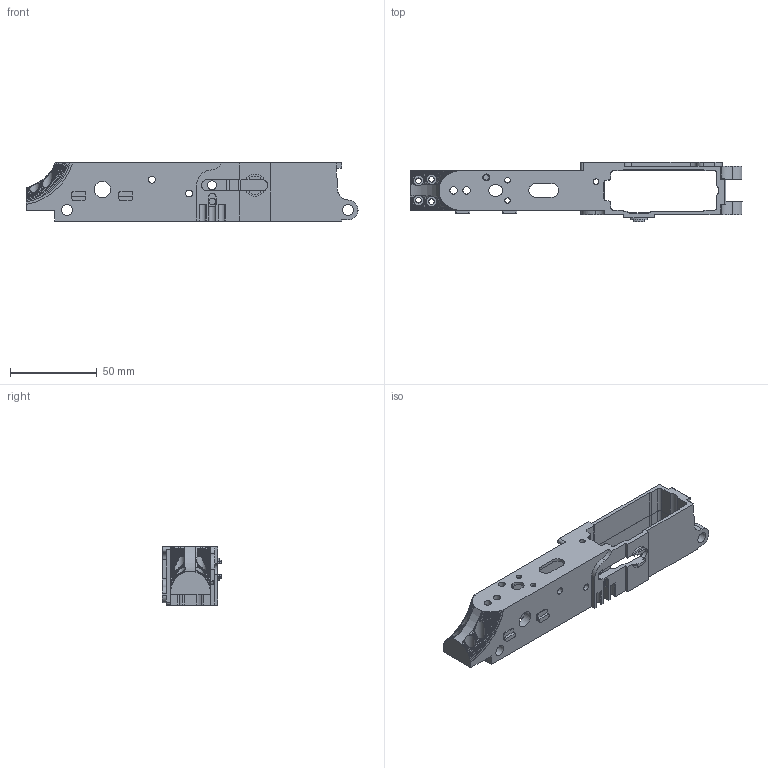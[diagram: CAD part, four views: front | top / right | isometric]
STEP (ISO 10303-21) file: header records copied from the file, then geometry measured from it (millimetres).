
FILE_DESCRIPTION(/* description */ (''),/* implementation_level */ '2;1');
FILE_NAME(/* name */ 'AR-00 Upper Lower.step',/* time_stamp */ '2022-01-15T13:05:13-06:00',/* author */ (''),/* organization */ (''),/* preprocessor_version */ 'ST-DEVELOPER v18.1',/* originating_system */ 'Autodesk Translation Framework v10.10.0.1391',/* authorisation */ '');
FILE_SCHEMA (('AUTOMOTIVE_DESIGN { 1 0 10303 214 3 1 1 }'));
Length unit declared in the file: inch
Products named in the file (1): AR-00 Upper Lower
Bounding box: 191.22 x 34.29 x 33.48 mm (x, y, z)
Volume: 51269.8 mm3; surface area: 35246.3 mm2
Topology: 1 solids, 1 shells, 508 faces, 1486 edges, 983 vertices
Faces by surface type: cylinder 273, plane 234, bspline 1
Full cylindrical faces by diameter (mm): 3.175 x3, 3.2 x5, 3.962 x6, 4.293 x2, 5.182 x1, 6 x4, 6.375 x4, 6.502 x1, 6.985 x1, 7.01 x1, 7.938 x1, 9.55 x2, 11.176 x1
Entity records: 17547 total; most frequent: CARTESIAN_POINT 3518, DIRECTION 3004, ORIENTED_EDGE 2972, EDGE_CURVE 1486, AXIS2_PLACEMENT_3D 1094, VERTEX_POINT 983, LINE 816, VECTOR 816
